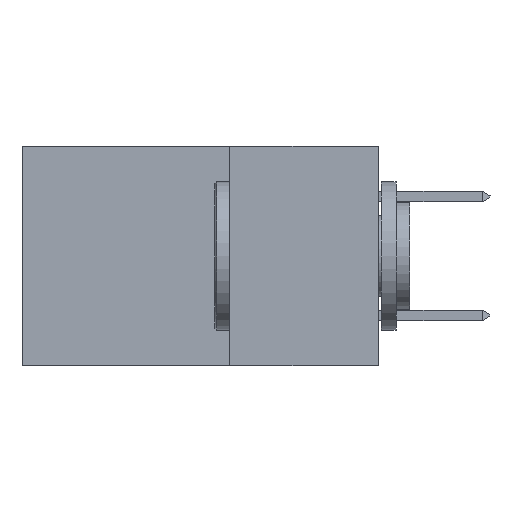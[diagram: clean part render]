
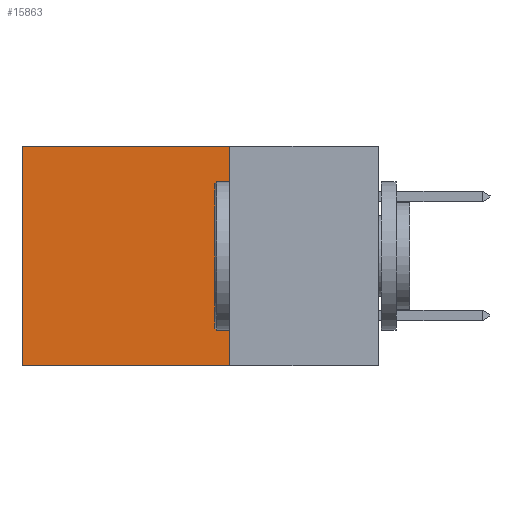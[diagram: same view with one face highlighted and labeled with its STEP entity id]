
A CAD part, left-side view. The second image highlights one B-rep face of the part: STEP entity #15863.
In plain terms, the highlighted planar face has unit normal (-1, 0, 0).
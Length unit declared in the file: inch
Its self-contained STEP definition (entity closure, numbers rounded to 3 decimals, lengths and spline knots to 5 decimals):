
#36 = CARTESIAN_POINT ( 'NONE',  ( 0.2615, 0.6, 0. ) ) ;
#289 = VERTEX_POINT ( 'NONE', #15274 ) ;
#1251 = VERTEX_POINT ( 'NONE', #11901 ) ;
#1529 = VECTOR ( 'NONE', #13141, 39.37008 ) ;
#1925 = EDGE_CURVE ( 'NONE', #289, #14889, #12931, .T. ) ;
#2540 = AXIS2_PLACEMENT_3D ( 'NONE', #9519, #18962, #10841 ) ;
#4320 = DIRECTION ( 'NONE',  ( 0., 0., -1. ) ) ;
#4556 = CARTESIAN_POINT ( 'NONE',  ( 0.2615, 0.6, -0.37 ) ) ;
#5716 = ORIENTED_EDGE ( 'NONE', *, *, #1925, .T. ) ;
#6594 = CARTESIAN_POINT ( 'NONE',  ( 0.2615, 0.25, 0. ) ) ;
#7000 = ORIENTED_EDGE ( 'NONE', *, *, #18755, .T. ) ;
#7076 = DIRECTION ( 'NONE',  ( 0., 1., 0. ) ) ;
#7649 = LINE ( 'NONE', #13806, #13121 ) ;
#8044 = VECTOR ( 'NONE', #7076, 39.37008 ) ;
#9519 = CARTESIAN_POINT ( 'NONE',  ( 0.2615, 0.25, -0.37 ) ) ;
#9663 = DIRECTION ( 'NONE',  ( 0., 0., -1. ) ) ;
#9945 = FACE_OUTER_BOUND ( 'NONE', #14872, .T. ) ;
#10195 = CARTESIAN_POINT ( 'NONE',  ( 0.2615, 0.25, -0.37 ) ) ;
#10841 = DIRECTION ( 'NONE',  ( 0., 0., -1. ) ) ;
#11370 = CARTESIAN_POINT ( 'NONE',  ( 0.2615, 0.6, -0.37 ) ) ;
#11901 = CARTESIAN_POINT ( 'NONE',  ( 0.2615, 0.25, -0.37 ) ) ;
#12403 = ORIENTED_EDGE ( 'NONE', *, *, #14725, .F. ) ;
#12510 = VECTOR ( 'NONE', #9663, 39.37008 ) ;
#12931 = LINE ( 'NONE', #6594, #1529 ) ;
#13121 = VECTOR ( 'NONE', #4320, 39.37008 ) ;
#13141 = DIRECTION ( 'NONE',  ( 0., 1., 0. ) ) ;
#13806 = CARTESIAN_POINT ( 'NONE',  ( 0.2615, 0.25, -0.37 ) ) ;
#14482 = ORIENTED_EDGE ( 'NONE', *, *, #18911, .F. ) ;
#14725 = EDGE_CURVE ( 'NONE', #289, #1251, #7649, .T. ) ;
#14870 = PLANE ( 'NONE',  #2540 ) ;
#14872 = EDGE_LOOP ( 'NONE', ( #7000, #14482, #12403, #5716 ) ) ;
#14889 = VERTEX_POINT ( 'NONE', #36 ) ;
#15274 = CARTESIAN_POINT ( 'NONE',  ( 0.2615, 0.25, 0. ) ) ;
#15863 = ADVANCED_FACE ( 'NONE', ( #9945 ), #14870, .F. ) ;
#17497 = LINE ( 'NONE', #11370, #12510 ) ;
#18755 = EDGE_CURVE ( 'NONE', #14889, #19641, #17497, .T. ) ;
#18911 = EDGE_CURVE ( 'NONE', #1251, #19641, #19709, .T. ) ;
#18962 = DIRECTION ( 'NONE',  ( 1., 0., 0. ) ) ;
#19641 = VERTEX_POINT ( 'NONE', #4556 ) ;
#19709 = LINE ( 'NONE', #10195, #8044 ) ;
